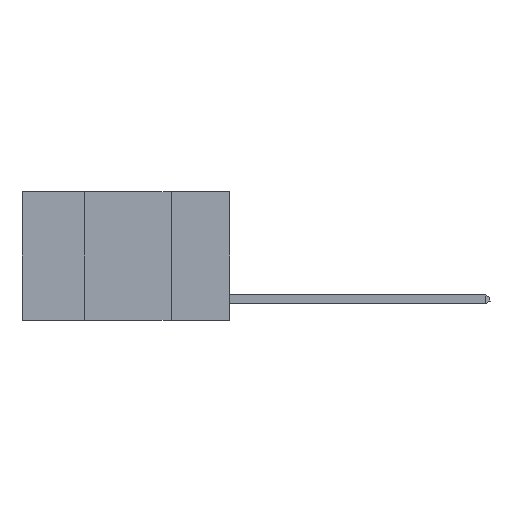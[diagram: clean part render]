
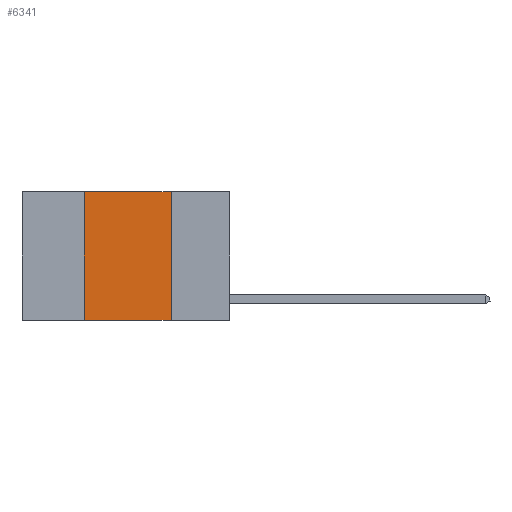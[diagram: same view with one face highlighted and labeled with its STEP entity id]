
A CAD part, left-side view. The second image highlights one B-rep face of the part: STEP entity #6341.
In plain terms, the highlighted planar face has unit normal (-1, 0, 0).
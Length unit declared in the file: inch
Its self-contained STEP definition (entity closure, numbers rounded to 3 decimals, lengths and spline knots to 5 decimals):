
#92 = VERTEX_POINT ( 'NONE', #539 ) ;
#539 = CARTESIAN_POINT ( 'NONE',  ( 0., 0.17, -0.37 ) ) ;
#816 = LINE ( 'NONE', #1614, #7549 ) ;
#1042 = DIRECTION ( 'NONE',  ( 1., 0., 0. ) ) ;
#1153 = ORIENTED_EDGE ( 'NONE', *, *, #7166, .T. ) ;
#1269 = LINE ( 'NONE', #4556, #9622 ) ;
#1358 = EDGE_CURVE ( 'NONE', #1428, #92, #816, .T. ) ;
#1365 = LINE ( 'NONE', #10426, #5331 ) ;
#1428 = VERTEX_POINT ( 'NONE', #9362 ) ;
#1490 = ORIENTED_EDGE ( 'NONE', *, *, #1358, .F. ) ;
#1614 = CARTESIAN_POINT ( 'NONE',  ( 0., 0.17, 0. ) ) ;
#1782 = DIRECTION ( 'NONE',  ( 0., 0., -1. ) ) ;
#1798 = DIRECTION ( 'NONE',  ( 0., 0., -1. ) ) ;
#1857 = DIRECTION ( 'NONE',  ( 0., -1., 0. ) ) ;
#1914 = FACE_OUTER_BOUND ( 'NONE', #6817, .T. ) ;
#2447 = EDGE_CURVE ( 'NONE', #9016, #1428, #1365, .T. ) ;
#2827 = CARTESIAN_POINT ( 'NONE',  ( 0., 0.6, 0. ) ) ;
#2939 = ORIENTED_EDGE ( 'NONE', *, *, #2447, .F. ) ;
#3420 = CARTESIAN_POINT ( 'NONE',  ( 0., 0.42, -0.37 ) ) ;
#3424 = VERTEX_POINT ( 'NONE', #3420 ) ;
#4048 = DIRECTION ( 'NONE',  ( 0., -1., 0. ) ) ;
#4556 = CARTESIAN_POINT ( 'NONE',  ( 0., 0.6, -0.37 ) ) ;
#5202 = PLANE ( 'NONE',  #5350 ) ;
#5331 = VECTOR ( 'NONE', #4048, 39.37008 ) ;
#5350 = AXIS2_PLACEMENT_3D ( 'NONE', #2827, #1042, #1798 ) ;
#5401 = VECTOR ( 'NONE', #8349, 39.37008 ) ;
#5903 = CARTESIAN_POINT ( 'NONE',  ( 0., 0.42, 0. ) ) ;
#6341 = ADVANCED_FACE ( 'NONE', ( #1914 ), #5202, .F. ) ;
#6733 = CARTESIAN_POINT ( 'NONE',  ( 0., 0.42, 0. ) ) ;
#6817 = EDGE_LOOP ( 'NONE', ( #1490, #2939, #7411, #1153 ) ) ;
#7166 = EDGE_CURVE ( 'NONE', #3424, #92, #1269, .T. ) ;
#7411 = ORIENTED_EDGE ( 'NONE', *, *, #9519, .F. ) ;
#7549 = VECTOR ( 'NONE', #1782, 39.37008 ) ;
#8349 = DIRECTION ( 'NONE',  ( 0., 0., 1. ) ) ;
#9016 = VERTEX_POINT ( 'NONE', #6733 ) ;
#9362 = CARTESIAN_POINT ( 'NONE',  ( 0., 0.17, 0. ) ) ;
#9519 = EDGE_CURVE ( 'NONE', #3424, #9016, #9959, .T. ) ;
#9622 = VECTOR ( 'NONE', #1857, 39.37008 ) ;
#9959 = LINE ( 'NONE', #5903, #5401 ) ;
#10426 = CARTESIAN_POINT ( 'NONE',  ( 0., 0.6, 0. ) ) ;
